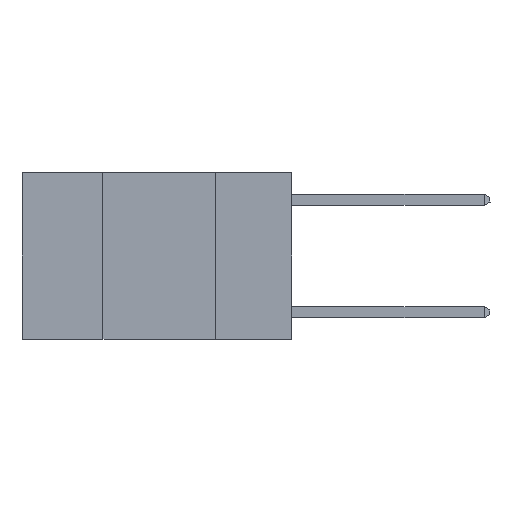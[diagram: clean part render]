
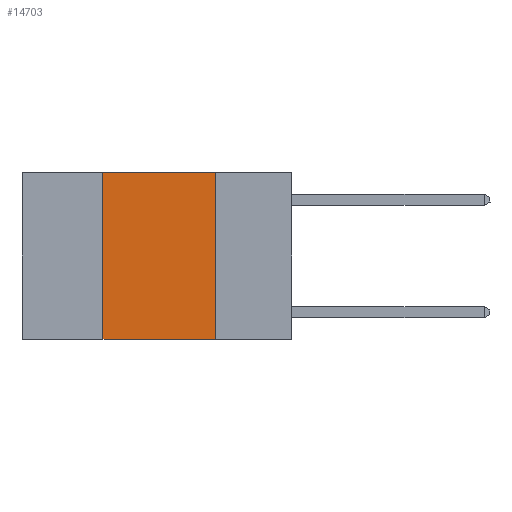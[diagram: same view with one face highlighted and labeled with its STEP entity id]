
A CAD part, left-side view. The second image highlights one B-rep face of the part: STEP entity #14703.
In plain terms, the highlighted planar face has unit normal (-1, 0, 0).
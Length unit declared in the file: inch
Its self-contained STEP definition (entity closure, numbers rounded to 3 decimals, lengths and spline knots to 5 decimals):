
#791 = CARTESIAN_POINT ( 'NONE',  ( 0., 0.6, 0. ) ) ;
#1193 = VERTEX_POINT ( 'NONE', #6719 ) ;
#1392 = CARTESIAN_POINT ( 'NONE',  ( 0., 0.6, 0. ) ) ;
#1405 = LINE ( 'NONE', #4196, #13579 ) ;
#1970 = EDGE_CURVE ( 'NONE', #7654, #1193, #11485, .T. ) ;
#2614 = DIRECTION ( 'NONE',  ( 1., 0., 0. ) ) ;
#2973 = CARTESIAN_POINT ( 'NONE',  ( 0., 0.6, -0.37 ) ) ;
#3614 = EDGE_CURVE ( 'NONE', #7654, #6634, #1405, .T. ) ;
#4196 = CARTESIAN_POINT ( 'NONE',  ( 0., 0.42, 0. ) ) ;
#4442 = EDGE_CURVE ( 'NONE', #6064, #1193, #13907, .T. ) ;
#4469 = CARTESIAN_POINT ( 'NONE',  ( 0., 0.42, 0. ) ) ;
#4693 = CARTESIAN_POINT ( 'NONE',  ( 0., 0.17, 0. ) ) ;
#5639 = EDGE_CURVE ( 'NONE', #6634, #6064, #8616, .T. ) ;
#6064 = VERTEX_POINT ( 'NONE', #9345 ) ;
#6634 = VERTEX_POINT ( 'NONE', #4469 ) ;
#6719 = CARTESIAN_POINT ( 'NONE',  ( 0., 0.17, -0.37 ) ) ;
#7467 = DIRECTION ( 'NONE',  ( 0., -1., 0. ) ) ;
#7557 = CARTESIAN_POINT ( 'NONE',  ( 0., 0.42, -0.37 ) ) ;
#7654 = VERTEX_POINT ( 'NONE', #7557 ) ;
#7736 = VECTOR ( 'NONE', #10575, 39.37008 ) ;
#7949 = AXIS2_PLACEMENT_3D ( 'NONE', #1392, #2614, #10871 ) ;
#8523 = PLANE ( 'NONE',  #7949 ) ;
#8616 = LINE ( 'NONE', #791, #10992 ) ;
#9119 = DIRECTION ( 'NONE',  ( 0., -1., 0. ) ) ;
#9345 = CARTESIAN_POINT ( 'NONE',  ( 0., 0.17, 0. ) ) ;
#9954 = EDGE_LOOP ( 'NONE', ( #14822, #10904, #12757, #14779 ) ) ;
#10575 = DIRECTION ( 'NONE',  ( 0., 0., -1. ) ) ;
#10871 = DIRECTION ( 'NONE',  ( 0., 0., -1. ) ) ;
#10904 = ORIENTED_EDGE ( 'NONE', *, *, #5639, .F. ) ;
#10992 = VECTOR ( 'NONE', #9119, 39.37008 ) ;
#11114 = VECTOR ( 'NONE', #7467, 39.37008 ) ;
#11485 = LINE ( 'NONE', #2973, #11114 ) ;
#12757 = ORIENTED_EDGE ( 'NONE', *, *, #3614, .F. ) ;
#13579 = VECTOR ( 'NONE', #14611, 39.37008 ) ;
#13907 = LINE ( 'NONE', #4693, #7736 ) ;
#14556 = FACE_OUTER_BOUND ( 'NONE', #9954, .T. ) ;
#14611 = DIRECTION ( 'NONE',  ( 0., 0., 1. ) ) ;
#14703 = ADVANCED_FACE ( 'NONE', ( #14556 ), #8523, .F. ) ;
#14779 = ORIENTED_EDGE ( 'NONE', *, *, #1970, .T. ) ;
#14822 = ORIENTED_EDGE ( 'NONE', *, *, #4442, .F. ) ;
